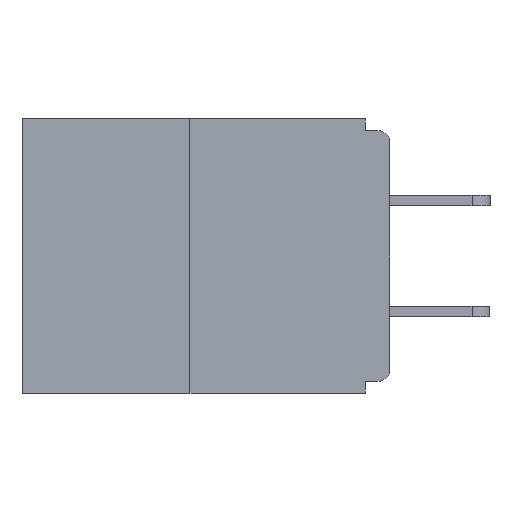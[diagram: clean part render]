
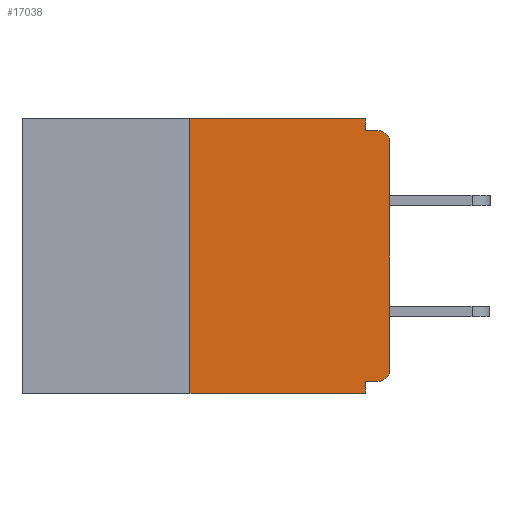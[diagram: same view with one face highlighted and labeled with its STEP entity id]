
A CAD part, left-side view. The second image highlights one B-rep face of the part: STEP entity #17038.
In plain terms, the highlighted planar face has unit normal (-1, 0, 0).
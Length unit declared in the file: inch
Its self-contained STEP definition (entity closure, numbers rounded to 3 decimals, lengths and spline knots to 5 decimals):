
#546 = LINE ( 'NONE', #11874, #3708 ) ;
#558 = VERTEX_POINT ( 'NONE', #17300 ) ;
#595 = CARTESIAN_POINT ( 'NONE',  ( 0., 0.031, 0. ) ) ;
#857 = AXIS2_PLACEMENT_3D ( 'NONE', #4733, #6060, #7466 ) ;
#1023 = DIRECTION ( 'NONE',  ( 0., 0., 1. ) ) ;
#1026 = EDGE_CURVE ( 'NONE', #15507, #14218, #7577, .T. ) ;
#1229 = LINE ( 'NONE', #5236, #2669 ) ;
#1388 = CARTESIAN_POINT ( 'NONE',  ( 0., 0.25, 0. ) ) ;
#1420 = CARTESIAN_POINT ( 'NONE',  ( 0., 0.46, 0. ) ) ;
#1538 = ORIENTED_EDGE ( 'NONE', *, *, #10714, .T. ) ;
#1753 = CARTESIAN_POINT ( 'NONE',  ( 0., 0., -0.313 ) ) ;
#1788 = CIRCLE ( 'NONE', #17045, 0.015 ) ;
#2220 = DIRECTION ( 'NONE',  ( 0., 0., -1. ) ) ;
#2370 = VERTEX_POINT ( 'NONE', #3169 ) ;
#2543 = ORIENTED_EDGE ( 'NONE', *, *, #9480, .F. ) ;
#2655 = AXIS2_PLACEMENT_3D ( 'NONE', #16750, #7541, #16625 ) ;
#2669 = VECTOR ( 'NONE', #8067, 39.37008 ) ;
#2841 = DIRECTION ( 'NONE',  ( 0., 1., 0. ) ) ;
#3169 = CARTESIAN_POINT ( 'NONE',  ( 0., 0., -0.03 ) ) ;
#3223 = ORIENTED_EDGE ( 'NONE', *, *, #10545, .T. ) ;
#3354 = EDGE_LOOP ( 'NONE', ( #13670, #2543, #8124, #5907, #14221, #4634, #1538, #3223, #4653, #16578 ) ) ;
#3363 = DIRECTION ( 'NONE',  ( 0., 0., 1. ) ) ;
#3708 = VECTOR ( 'NONE', #1023, 39.37008 ) ;
#3796 = LINE ( 'NONE', #15140, #12495 ) ;
#4122 = CARTESIAN_POINT ( 'NONE',  ( 0., 0.031, -0.343 ) ) ;
#4440 = CIRCLE ( 'NONE', #857, 0.015 ) ;
#4634 = ORIENTED_EDGE ( 'NONE', *, *, #13873, .T. ) ;
#4653 = ORIENTED_EDGE ( 'NONE', *, *, #8997, .F. ) ;
#4733 = CARTESIAN_POINT ( 'NONE',  ( 0., 0.015, -0.313 ) ) ;
#5236 = CARTESIAN_POINT ( 'NONE',  ( 0., 0., -0.015 ) ) ;
#5430 = DIRECTION ( 'NONE',  ( 0., 0., -1. ) ) ;
#5907 = ORIENTED_EDGE ( 'NONE', *, *, #16886, .F. ) ;
#5910 = EDGE_CURVE ( 'NONE', #6457, #10565, #9206, .T. ) ;
#6060 = DIRECTION ( 'NONE',  ( -1., 0., 0. ) ) ;
#6377 = VECTOR ( 'NONE', #2841, 39.37008 ) ;
#6390 = VECTOR ( 'NONE', #13586, 39.37008 ) ;
#6457 = VERTEX_POINT ( 'NONE', #9611 ) ;
#7269 = DIRECTION ( 'NONE',  ( 0., -1., 0. ) ) ;
#7370 = CARTESIAN_POINT ( 'NONE',  ( 0., 0.031, -0.015 ) ) ;
#7466 = DIRECTION ( 'NONE',  ( 0., 0., -1. ) ) ;
#7541 = DIRECTION ( 'NONE',  ( 1., 0., 0. ) ) ;
#7577 = LINE ( 'NONE', #595, #12279 ) ;
#7586 = CARTESIAN_POINT ( 'NONE',  ( 0., 0.25, -0.343 ) ) ;
#8067 = DIRECTION ( 'NONE',  ( 0., -1., 0. ) ) ;
#8124 = ORIENTED_EDGE ( 'NONE', *, *, #8575, .T. ) ;
#8417 = VECTOR ( 'NONE', #3363, 39.37008 ) ;
#8575 = EDGE_CURVE ( 'NONE', #8742, #13760, #3796, .T. ) ;
#8742 = VERTEX_POINT ( 'NONE', #7586 ) ;
#8765 = CARTESIAN_POINT ( 'NONE',  ( 0., 0.25, 0. ) ) ;
#8997 = EDGE_CURVE ( 'NONE', #14218, #558, #1229, .T. ) ;
#9018 = CARTESIAN_POINT ( 'NONE',  ( 0., 0.031, -0.328 ) ) ;
#9206 = LINE ( 'NONE', #16463, #6377 ) ;
#9480 = EDGE_CURVE ( 'NONE', #8742, #13424, #12044, .T. ) ;
#9611 = CARTESIAN_POINT ( 'NONE',  ( 0., 0.015, -0.328 ) ) ;
#9673 = LINE ( 'NONE', #1420, #6390 ) ;
#10545 = EDGE_CURVE ( 'NONE', #2370, #558, #1788, .T. ) ;
#10565 = VERTEX_POINT ( 'NONE', #9018 ) ;
#10714 = EDGE_CURVE ( 'NONE', #15892, #2370, #546, .T. ) ;
#10847 = EDGE_CURVE ( 'NONE', #13424, #15507, #9673, .T. ) ;
#11874 = CARTESIAN_POINT ( 'NONE',  ( 0., 0., 0. ) ) ;
#12044 = LINE ( 'NONE', #8765, #8417 ) ;
#12279 = VECTOR ( 'NONE', #16763, 39.37008 ) ;
#12495 = VECTOR ( 'NONE', #7269, 39.37008 ) ;
#13072 = LINE ( 'NONE', #4122, #13278 ) ;
#13228 = DIRECTION ( 'NONE',  ( -1., 0., 0. ) ) ;
#13278 = VECTOR ( 'NONE', #5430, 39.37008 ) ;
#13424 = VERTEX_POINT ( 'NONE', #1388 ) ;
#13586 = DIRECTION ( 'NONE',  ( 0., -1., 0. ) ) ;
#13670 = ORIENTED_EDGE ( 'NONE', *, *, #10847, .F. ) ;
#13688 = FACE_OUTER_BOUND ( 'NONE', #3354, .T. ) ;
#13760 = VERTEX_POINT ( 'NONE', #15308 ) ;
#13873 = EDGE_CURVE ( 'NONE', #6457, #15892, #4440, .T. ) ;
#14178 = CARTESIAN_POINT ( 'NONE',  ( 0., 0.031, 0. ) ) ;
#14218 = VERTEX_POINT ( 'NONE', #7370 ) ;
#14221 = ORIENTED_EDGE ( 'NONE', *, *, #5910, .F. ) ;
#15140 = CARTESIAN_POINT ( 'NONE',  ( 0., 0.46, -0.343 ) ) ;
#15308 = CARTESIAN_POINT ( 'NONE',  ( 0., 0.031, -0.343 ) ) ;
#15507 = VERTEX_POINT ( 'NONE', #14178 ) ;
#15664 = PLANE ( 'NONE',  #2655 ) ;
#15792 = CARTESIAN_POINT ( 'NONE',  ( 0., 0.015, -0.03 ) ) ;
#15892 = VERTEX_POINT ( 'NONE', #1753 ) ;
#16463 = CARTESIAN_POINT ( 'NONE',  ( 0., 0., -0.328 ) ) ;
#16578 = ORIENTED_EDGE ( 'NONE', *, *, #1026, .F. ) ;
#16625 = DIRECTION ( 'NONE',  ( 0., 0., -1. ) ) ;
#16750 = CARTESIAN_POINT ( 'NONE',  ( 0., 0.46, 0. ) ) ;
#16763 = DIRECTION ( 'NONE',  ( 0., 0., -1. ) ) ;
#16886 = EDGE_CURVE ( 'NONE', #10565, #13760, #13072, .T. ) ;
#17038 = ADVANCED_FACE ( 'NONE', ( #13688 ), #15664, .F. ) ;
#17045 = AXIS2_PLACEMENT_3D ( 'NONE', #15792, #13228, #2220 ) ;
#17300 = CARTESIAN_POINT ( 'NONE',  ( 0., 0.015, -0.015 ) ) ;
